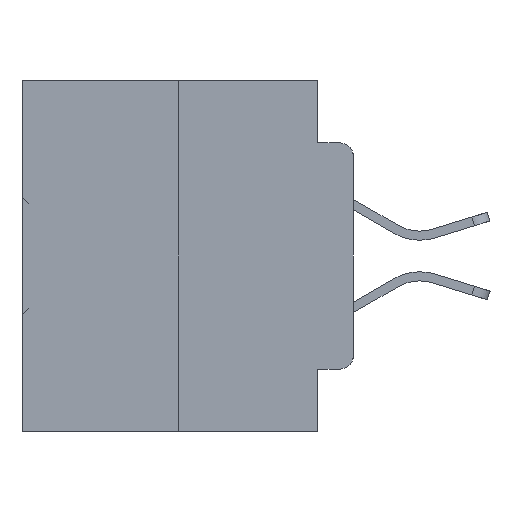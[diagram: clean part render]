
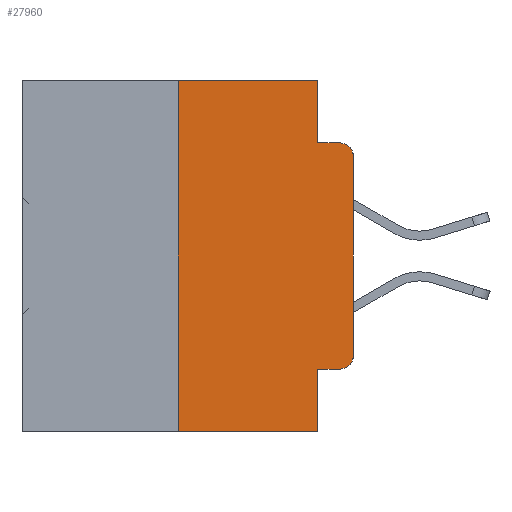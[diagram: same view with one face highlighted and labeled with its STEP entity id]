
A CAD part, left-side view. The second image highlights one B-rep face of the part: STEP entity #27960.
In plain terms, the highlighted planar face has unit normal (-1, 0, 0).
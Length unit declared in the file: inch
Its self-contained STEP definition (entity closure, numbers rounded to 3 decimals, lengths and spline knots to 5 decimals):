
#343 = VECTOR ( 'NONE', #36376, 39.37008 ) ;
#498 = CARTESIAN_POINT ( 'NONE',  ( 0., 0., -0.1085 ) ) ;
#1312 = LINE ( 'NONE', #34761, #30820 ) ;
#2256 = DIRECTION ( 'NONE',  ( 0., 0., -1. ) ) ;
#2626 = ORIENTED_EDGE ( 'NONE', *, *, #25600, .T. ) ;
#2811 = PLANE ( 'NONE',  #4908 ) ;
#3249 = VECTOR ( 'NONE', #27255, 39.37008 ) ;
#3670 = DIRECTION ( 'NONE',  ( 0., 0., -1. ) ) ;
#4064 = CARTESIAN_POINT ( 'NONE',  ( 0., 0.02, -0.0885 ) ) ;
#4908 = AXIS2_PLACEMENT_3D ( 'NONE', #8401, #17078, #2256 ) ;
#6156 = CARTESIAN_POINT ( 'NONE',  ( 0., 0.473, -0.5 ) ) ;
#6566 = AXIS2_PLACEMENT_3D ( 'NONE', #9613, #26842, #32269 ) ;
#7107 = CARTESIAN_POINT ( 'NONE',  ( 0., 0.473, 0. ) ) ;
#7113 = EDGE_CURVE ( 'NONE', #11399, #15281, #22518, .T. ) ;
#7607 = EDGE_CURVE ( 'NONE', #11399, #10959, #32325, .T. ) ;
#7785 = LINE ( 'NONE', #33031, #3249 ) ;
#8401 = CARTESIAN_POINT ( 'NONE',  ( 0., 0.473, 0. ) ) ;
#8584 = FACE_OUTER_BOUND ( 'NONE', #30448, .T. ) ;
#9327 = ORIENTED_EDGE ( 'NONE', *, *, #23910, .F. ) ;
#9611 = DIRECTION ( 'NONE',  ( -1., 0., 0. ) ) ;
#9613 = CARTESIAN_POINT ( 'NONE',  ( 0., 0.02, -0.1085 ) ) ;
#9678 = EDGE_CURVE ( 'NONE', #11426, #10959, #31512, .T. ) ;
#10959 = VERTEX_POINT ( 'NONE', #23146 ) ;
#11081 = VERTEX_POINT ( 'NONE', #19171 ) ;
#11399 = VERTEX_POINT ( 'NONE', #23959 ) ;
#11426 = VERTEX_POINT ( 'NONE', #34978 ) ;
#11669 = AXIS2_PLACEMENT_3D ( 'NONE', #22591, #9611, #34878 ) ;
#12942 = ORIENTED_EDGE ( 'NONE', *, *, #7113, .F. ) ;
#14843 = ORIENTED_EDGE ( 'NONE', *, *, #17007, .F. ) ;
#15281 = VERTEX_POINT ( 'NONE', #34241 ) ;
#15347 = DIRECTION ( 'NONE',  ( 0., -1., 0. ) ) ;
#15530 = CARTESIAN_POINT ( 'NONE',  ( 0., 0.051, -0.0885 ) ) ;
#16378 = ORIENTED_EDGE ( 'NONE', *, *, #20250, .T. ) ;
#17007 = EDGE_CURVE ( 'NONE', #28337, #22343, #24983, .T. ) ;
#17078 = DIRECTION ( 'NONE',  ( 1., 0., 0. ) ) ;
#18130 = ORIENTED_EDGE ( 'NONE', *, *, #9678, .F. ) ;
#18365 = CARTESIAN_POINT ( 'NONE',  ( 0., 0.051, 0. ) ) ;
#18629 = VERTEX_POINT ( 'NONE', #4064 ) ;
#18661 = EDGE_CURVE ( 'NONE', #32239, #29304, #7785, .T. ) ;
#19171 = CARTESIAN_POINT ( 'NONE',  ( 0., 0.02, -0.4115 ) ) ;
#19269 = CARTESIAN_POINT ( 'NONE',  ( 0., 0.051, 0. ) ) ;
#19592 = CIRCLE ( 'NONE', #6566, 0.02 ) ;
#20250 = EDGE_CURVE ( 'NONE', #11081, #32239, #20538, .T. ) ;
#20538 = CIRCLE ( 'NONE', #11669, 0.02 ) ;
#20554 = CARTESIAN_POINT ( 'NONE',  ( 0., 0., -0.3915 ) ) ;
#21164 = DIRECTION ( 'NONE',  ( 0., -1., 0. ) ) ;
#22150 = VECTOR ( 'NONE', #28289, 39.37008 ) ;
#22343 = VERTEX_POINT ( 'NONE', #36678 ) ;
#22518 = LINE ( 'NONE', #33870, #22150 ) ;
#22591 = CARTESIAN_POINT ( 'NONE',  ( 0., 0.02, -0.3915 ) ) ;
#23146 = CARTESIAN_POINT ( 'NONE',  ( 0., 0.051, -0.5 ) ) ;
#23295 = ORIENTED_EDGE ( 'NONE', *, *, #18661, .T. ) ;
#23910 = EDGE_CURVE ( 'NONE', #15281, #28337, #24324, .T. ) ;
#23959 = CARTESIAN_POINT ( 'NONE',  ( 0., 0.25, -0.5 ) ) ;
#24153 = ORIENTED_EDGE ( 'NONE', *, *, #30336, .T. ) ;
#24324 = LINE ( 'NONE', #7107, #34326 ) ;
#24983 = LINE ( 'NONE', #18365, #343 ) ;
#25515 = EDGE_CURVE ( 'NONE', #22343, #18629, #26665, .T. ) ;
#25600 = EDGE_CURVE ( 'NONE', #29304, #18629, #19592, .T. ) ;
#26482 = VECTOR ( 'NONE', #3670, 39.37008 ) ;
#26665 = LINE ( 'NONE', #15530, #28452 ) ;
#26842 = DIRECTION ( 'NONE',  ( -1., 0., 0. ) ) ;
#27255 = DIRECTION ( 'NONE',  ( 0., 0., 1. ) ) ;
#27960 = ADVANCED_FACE ( 'NONE', ( #8584 ), #2811, .F. ) ;
#28289 = DIRECTION ( 'NONE',  ( 0., 0., 1. ) ) ;
#28337 = VERTEX_POINT ( 'NONE', #19269 ) ;
#28452 = VECTOR ( 'NONE', #15347, 39.37008 ) ;
#29101 = CARTESIAN_POINT ( 'NONE',  ( 0., 0.051, 0. ) ) ;
#29304 = VERTEX_POINT ( 'NONE', #498 ) ;
#29925 = ORIENTED_EDGE ( 'NONE', *, *, #25515, .F. ) ;
#29929 = VECTOR ( 'NONE', #31763, 39.37008 ) ;
#30336 = EDGE_CURVE ( 'NONE', #11426, #11081, #1312, .T. ) ;
#30448 = EDGE_LOOP ( 'NONE', ( #23295, #2626, #29925, #14843, #9327, #12942, #31900, #18130, #24153, #16378 ) ) ;
#30820 = VECTOR ( 'NONE', #34567, 39.37008 ) ;
#31512 = LINE ( 'NONE', #29101, #26482 ) ;
#31763 = DIRECTION ( 'NONE',  ( 0., -1., 0. ) ) ;
#31900 = ORIENTED_EDGE ( 'NONE', *, *, #7607, .T. ) ;
#32239 = VERTEX_POINT ( 'NONE', #20554 ) ;
#32269 = DIRECTION ( 'NONE',  ( 0., 0., -1. ) ) ;
#32325 = LINE ( 'NONE', #6156, #29929 ) ;
#33031 = CARTESIAN_POINT ( 'NONE',  ( 0., 0., 0. ) ) ;
#33870 = CARTESIAN_POINT ( 'NONE',  ( 0., 0.25, 0. ) ) ;
#34241 = CARTESIAN_POINT ( 'NONE',  ( 0., 0.25, 0. ) ) ;
#34326 = VECTOR ( 'NONE', #21164, 39.37008 ) ;
#34567 = DIRECTION ( 'NONE',  ( 0., -1., 0. ) ) ;
#34761 = CARTESIAN_POINT ( 'NONE',  ( 0., 0.051, -0.4115 ) ) ;
#34878 = DIRECTION ( 'NONE',  ( 0., 0., -1. ) ) ;
#34978 = CARTESIAN_POINT ( 'NONE',  ( 0., 0.051, -0.4115 ) ) ;
#36376 = DIRECTION ( 'NONE',  ( 0., 0., -1. ) ) ;
#36678 = CARTESIAN_POINT ( 'NONE',  ( 0., 0.051, -0.0885 ) ) ;
